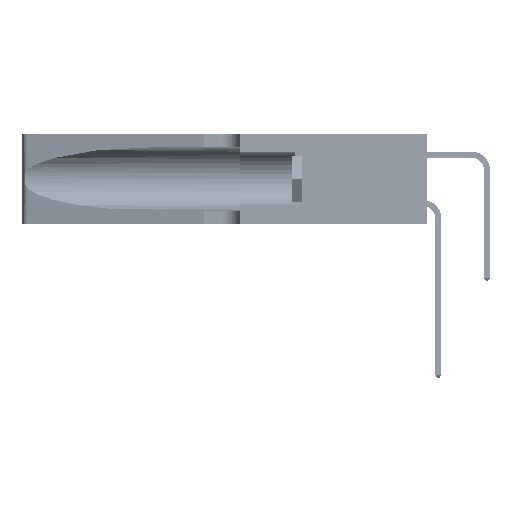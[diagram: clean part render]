
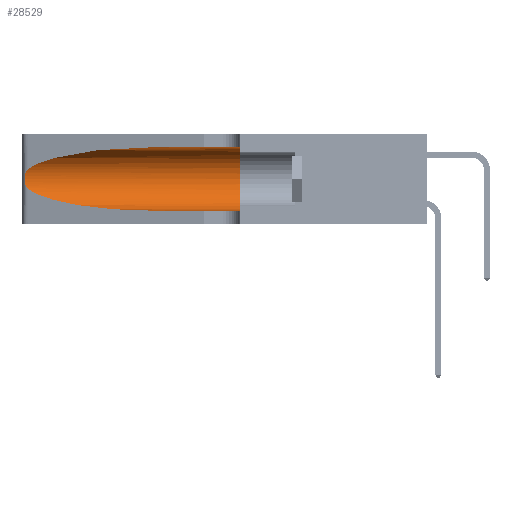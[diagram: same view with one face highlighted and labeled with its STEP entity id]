
A CAD part, left-side view. The second image highlights one B-rep face of the part: STEP entity #28529.
In plain terms, the highlighted cylindrical face has radius 3.308 mm (diameter 6.617 mm), a partial arc.
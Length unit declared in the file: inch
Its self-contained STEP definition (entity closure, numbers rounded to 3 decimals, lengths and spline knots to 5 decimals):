
#303 = CARTESIAN_POINT ( 'NONE',  ( 0.18966, 0.96281, 0.31525 ) ) ;
#1631 = CARTESIAN_POINT ( 'NONE',  ( 0.26017, 1.23833, 0.17102 ) ) ;
#2212 = CARTESIAN_POINT ( 'NONE',  ( 0.1305, 1.61858, 0.05475 ) ) ;
#2390 =( BOUNDED_CURVE ( )  B_SPLINE_CURVE ( 3, ( #11670, #303, #26723, #4186 ),
 .UNSPECIFIED., .F., .F. ) 
 B_SPLINE_CURVE_WITH_KNOTS ( ( 4, 4 ),
 ( 1.5708, 2.84003 ),
 .UNSPECIFIED. ) 
 CURVE ( )  GEOMETRIC_REPRESENTATION_ITEM ( )  RATIONAL_B_SPLINE_CURVE ( ( 1., 0.87, 0.87, 1. ) ) 
 REPRESENTATION_ITEM ( '' )  );
#3679 = EDGE_CURVE ( 'NONE', #5709, #3682, #18470, .T. ) ;
#3682 = VERTEX_POINT ( 'NONE', #16860 ) ;
#4186 = CARTESIAN_POINT ( 'NONE',  ( 0.25487, 1.22718, 0.22369 ) ) ;
#4629 = ORIENTED_EDGE ( 'NONE', *, *, #9519, .T. ) ;
#5471 = CARTESIAN_POINT ( 'NONE',  ( 0.25789, 1.23486, 0.15765 ) ) ;
#5709 = VERTEX_POINT ( 'NONE', #19617 ) ;
#7364 = EDGE_LOOP ( 'NONE', ( #11092, #15830, #4629, #23033, #13556, #30615 ) ) ;
#7819 = VERTEX_POINT ( 'NONE', #9085 ) ;
#9085 = CARTESIAN_POINT ( 'NONE',  ( 0.1305, 0.72297, 0.05475 ) ) ;
#9107 = CARTESIAN_POINT ( 'NONE',  ( 0.25555, 1.22994, 0.2215 ) ) ;
#9274 = CARTESIAN_POINT ( 'NONE',  ( 0.25555, 1.22993, 0.14849 ) ) ;
#9519 = EDGE_CURVE ( 'NONE', #3682, #7819, #9721, .T. ) ;
#9721 =( BOUNDED_CURVE ( )  B_SPLINE_CURVE ( 3, ( #27462, #19933, #34951, #12582 ),
 .UNSPECIFIED., .F., .F. ) 
 B_SPLINE_CURVE_WITH_KNOTS ( ( 4, 4 ),
 ( 3.44316, 4.71239 ),
 .UNSPECIFIED. ) 
 CURVE ( )  GEOMETRIC_REPRESENTATION_ITEM ( )  RATIONAL_B_SPLINE_CURVE ( ( 1., 0.87, 0.87, 1. ) ) 
 REPRESENTATION_ITEM ( '' )  );
#10534 = DIRECTION ( 'NONE',  ( 0., 0., -1. ) ) ;
#10778 = LINE ( 'NONE', #2212, #20752 ) ;
#11092 = ORIENTED_EDGE ( 'NONE', *, *, #42116, .T. ) ;
#11670 = CARTESIAN_POINT ( 'NONE',  ( 0.1305, 0.72297, 0.31525 ) ) ;
#12582 = CARTESIAN_POINT ( 'NONE',  ( 0.1305, 0.72297, 0.05475 ) ) ;
#13556 = ORIENTED_EDGE ( 'NONE', *, *, #27892, .F. ) ;
#15310 = CARTESIAN_POINT ( 'NONE',  ( 0.1305, 0.35, 0.31525 ) ) ;
#15830 = ORIENTED_EDGE ( 'NONE', *, *, #3679, .T. ) ;
#16714 = CARTESIAN_POINT ( 'NONE',  ( 0.25787, 1.23484, 0.2124 ) ) ;
#16860 = CARTESIAN_POINT ( 'NONE',  ( 0.25487, 1.22718, 0.14631 ) ) ;
#18470 = B_SPLINE_CURVE_WITH_KNOTS ( 'NONE', 3,
 ( #39081, #9107, #42502, #16714, #42835, #20440, #46588, #24207, #1631, #27957, #5471, #31728, #9274, #35481 ),
 .UNSPECIFIED., .F., .F.,
 ( 4, 2, 2, 2, 2, 2, 4 ),
 ( 0., 0.00027, 0.00053, 0.00107, 0.0016, 0.00187, 0.00214 ),
 .UNSPECIFIED. ) ;
#18899 = CARTESIAN_POINT ( 'NONE',  ( 0.1305, 0.35, 0.05475 ) ) ;
#19617 = CARTESIAN_POINT ( 'NONE',  ( 0.25487, 1.22718, 0.22369 ) ) ;
#19933 = CARTESIAN_POINT ( 'NONE',  ( 0.2373, 1.15595, 0.08982 ) ) ;
#20299 = VERTEX_POINT ( 'NONE', #31980 ) ;
#20440 = CARTESIAN_POINT ( 'NONE',  ( 0.26018, 1.23835, 0.19895 ) ) ;
#20752 = VECTOR ( 'NONE', #32315, 39.37008 ) ;
#21400 = CARTESIAN_POINT ( 'NONE',  ( 0.1305, 0.35, 0.185 ) ) ;
#22662 = AXIS2_PLACEMENT_3D ( 'NONE', #29170, #32956, #10534 ) ;
#22689 = DIRECTION ( 'NONE',  ( 0., -1., 0. ) ) ;
#23033 = ORIENTED_EDGE ( 'NONE', *, *, #39831, .T. ) ;
#23664 = VERTEX_POINT ( 'NONE', #15310 ) ;
#24207 = CARTESIAN_POINT ( 'NONE',  ( 0.26075, 1.23896, 0.178 ) ) ;
#24808 = EDGE_CURVE ( 'NONE', #20299, #23664, #37532, .T. ) ;
#25144 = DIRECTION ( 'NONE',  ( 0., 0., 1. ) ) ;
#26723 = CARTESIAN_POINT ( 'NONE',  ( 0.2373, 1.15595, 0.28018 ) ) ;
#27462 = CARTESIAN_POINT ( 'NONE',  ( 0.25487, 1.22718, 0.14631 ) ) ;
#27892 = EDGE_CURVE ( 'NONE', #23664, #40116, #37331, .T. ) ;
#27920 = FACE_OUTER_BOUND ( 'NONE', #7364, .T. ) ;
#27957 = CARTESIAN_POINT ( 'NONE',  ( 0.25856, 1.23593, 0.16098 ) ) ;
#28529 = ADVANCED_FACE ( 'NONE', ( #27920 ), #45425, .F. ) ;
#29170 = CARTESIAN_POINT ( 'NONE',  ( 0.1305, 1.61858, 0.185 ) ) ;
#30615 = ORIENTED_EDGE ( 'NONE', *, *, #24808, .F. ) ;
#31728 = CARTESIAN_POINT ( 'NONE',  ( 0.25639, 1.23186, 0.15144 ) ) ;
#31980 = CARTESIAN_POINT ( 'NONE',  ( 0.1305, 0.72297, 0.31525 ) ) ;
#32315 = DIRECTION ( 'NONE',  ( 0., -1., 0. ) ) ;
#32956 = DIRECTION ( 'NONE',  ( 0., -1., 0. ) ) ;
#34507 = AXIS2_PLACEMENT_3D ( 'NONE', #21400, #47509, #25144 ) ;
#34951 = CARTESIAN_POINT ( 'NONE',  ( 0.18966, 0.96281, 0.05475 ) ) ;
#35190 = VECTOR ( 'NONE', #22689, 39.37008 ) ;
#35481 = CARTESIAN_POINT ( 'NONE',  ( 0.25487, 1.22718, 0.14631 ) ) ;
#37331 = CIRCLE ( 'NONE', #34507, 0.13025 ) ;
#37532 = LINE ( 'NONE', #41263, #35190 ) ;
#39081 = CARTESIAN_POINT ( 'NONE',  ( 0.25487, 1.22718, 0.22369 ) ) ;
#39831 = EDGE_CURVE ( 'NONE', #7819, #40116, #10778, .T. ) ;
#40116 = VERTEX_POINT ( 'NONE', #18899 ) ;
#41263 = CARTESIAN_POINT ( 'NONE',  ( 0.1305, 1.61858, 0.31525 ) ) ;
#42116 = EDGE_CURVE ( 'NONE', #20299, #5709, #2390, .T. ) ;
#42502 = CARTESIAN_POINT ( 'NONE',  ( 0.25639, 1.23184, 0.21858 ) ) ;
#42835 = CARTESIAN_POINT ( 'NONE',  ( 0.25854, 1.2359, 0.20912 ) ) ;
#45425 = CYLINDRICAL_SURFACE ( 'NONE', #22662, 0.13025 ) ;
#46588 = CARTESIAN_POINT ( 'NONE',  ( 0.26075, 1.23896, 0.19203 ) ) ;
#47509 = DIRECTION ( 'NONE',  ( 0., 1., 0. ) ) ;
